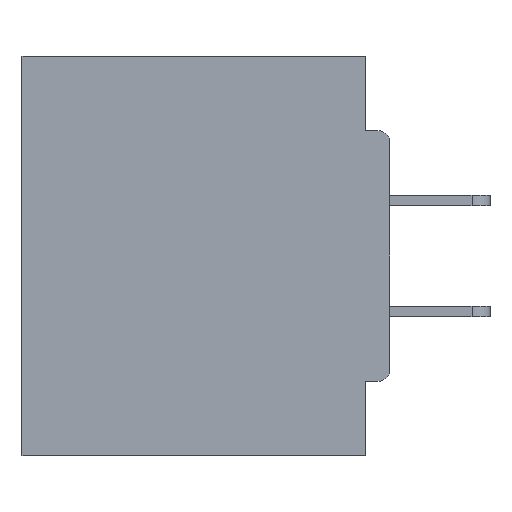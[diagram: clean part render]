
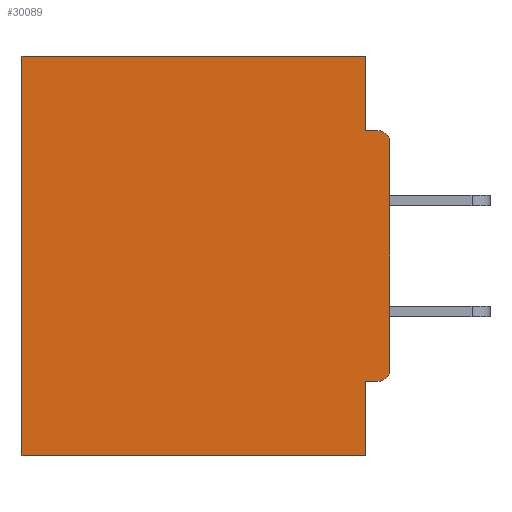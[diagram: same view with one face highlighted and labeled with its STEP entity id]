
A CAD part, left-side view. The second image highlights one B-rep face of the part: STEP entity #30089.
In plain terms, the highlighted planar face has unit normal (-1, 0, 0).
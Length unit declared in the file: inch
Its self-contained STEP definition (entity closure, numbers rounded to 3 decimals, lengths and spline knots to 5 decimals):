
#59 = ORIENTED_EDGE ( 'NONE', *, *, #22481, .F. ) ;
#153 = CIRCLE ( 'NONE', #36718, 0.015 ) ;
#462 = VERTEX_POINT ( 'NONE', #21627 ) ;
#936 = EDGE_CURVE ( 'NONE', #9909, #26018, #36658, .T. ) ;
#1723 = ORIENTED_EDGE ( 'NONE', *, *, #35162, .F. ) ;
#2313 = VECTOR ( 'NONE', #24132, 39.37008 ) ;
#2850 = CARTESIAN_POINT ( 'NONE',  ( 0.298, 0.015, -0.1085 ) ) ;
#4023 = DIRECTION ( 'NONE',  ( 0., 1., 0. ) ) ;
#4083 = CARTESIAN_POINT ( 'NONE',  ( 0.298, 0., 0. ) ) ;
#4333 = CIRCLE ( 'NONE', #4346, 0.015 ) ;
#4346 = AXIS2_PLACEMENT_3D ( 'NONE', #2850, #21541, #33391 ) ;
#4539 = ORIENTED_EDGE ( 'NONE', *, *, #19001, .T. ) ;
#4568 = LINE ( 'NONE', #33875, #5069 ) ;
#4732 = VECTOR ( 'NONE', #34768, 39.37008 ) ;
#4946 = FACE_OUTER_BOUND ( 'NONE', #10687, .T. ) ;
#5069 = VECTOR ( 'NONE', #34135, 39.37008 ) ;
#5492 = ORIENTED_EDGE ( 'NONE', *, *, #33387, .F. ) ;
#7512 = CARTESIAN_POINT ( 'NONE',  ( 0.298, 0.031, 0. ) ) ;
#7605 = AXIS2_PLACEMENT_3D ( 'NONE', #20560, #32809, #38469 ) ;
#7866 = VECTOR ( 'NONE', #4023, 39.37008 ) ;
#8174 = ORIENTED_EDGE ( 'NONE', *, *, #10169, .T. ) ;
#8887 = VECTOR ( 'NONE', #9446, 39.37008 ) ;
#9446 = DIRECTION ( 'NONE',  ( 0., 0., -1. ) ) ;
#9909 = VERTEX_POINT ( 'NONE', #7512 ) ;
#10169 = EDGE_CURVE ( 'NONE', #17332, #36294, #153, .T. ) ;
#10347 = DIRECTION ( 'NONE',  ( 0., 1., 0. ) ) ;
#10687 = EDGE_LOOP ( 'NONE', ( #37894, #35037, #59, #37771, #4539, #27794, #1723, #27116, #8174, #5492 ) ) ;
#12202 = VERTEX_POINT ( 'NONE', #34867 ) ;
#13095 = LINE ( 'NONE', #13332, #7866 ) ;
#13332 = CARTESIAN_POINT ( 'NONE',  ( 0.298, 0., -0.5 ) ) ;
#13822 = CARTESIAN_POINT ( 'NONE',  ( 0.298, 0., 0. ) ) ;
#13982 = EDGE_CURVE ( 'NONE', #462, #27365, #24177, .T. ) ;
#14369 = VECTOR ( 'NONE', #31480, 39.37008 ) ;
#15449 = CARTESIAN_POINT ( 'NONE',  ( 0.298, 0.46, 0. ) ) ;
#16356 = LINE ( 'NONE', #27222, #34872 ) ;
#17087 = LINE ( 'NONE', #13822, #4732 ) ;
#17332 = VERTEX_POINT ( 'NONE', #32124 ) ;
#19001 = EDGE_CURVE ( 'NONE', #26018, #21283, #16356, .T. ) ;
#19309 = VERTEX_POINT ( 'NONE', #31864 ) ;
#19492 = CARTESIAN_POINT ( 'NONE',  ( 0.298, 0., -0.4065 ) ) ;
#20560 = CARTESIAN_POINT ( 'NONE',  ( 0.298, 0., 0. ) ) ;
#21283 = VERTEX_POINT ( 'NONE', #28031 ) ;
#21541 = DIRECTION ( 'NONE',  ( -1., 0., 0. ) ) ;
#21627 = CARTESIAN_POINT ( 'NONE',  ( 0.298, 0.031, -0.0935 ) ) ;
#22481 = EDGE_CURVE ( 'NONE', #9909, #462, #32698, .T. ) ;
#24132 = DIRECTION ( 'NONE',  ( 0., -1., 0. ) ) ;
#24177 = LINE ( 'NONE', #38956, #2313 ) ;
#24803 = CARTESIAN_POINT ( 'NONE',  ( 0.298, 0., -0.1085 ) ) ;
#26018 = VERTEX_POINT ( 'NONE', #15449 ) ;
#26564 = LINE ( 'NONE', #19492, #35992 ) ;
#27116 = ORIENTED_EDGE ( 'NONE', *, *, #28807, .F. ) ;
#27187 = CARTESIAN_POINT ( 'NONE',  ( 0.298, 0.015, -0.3915 ) ) ;
#27222 = CARTESIAN_POINT ( 'NONE',  ( 0.298, 0.46, 0. ) ) ;
#27365 = VERTEX_POINT ( 'NONE', #33293 ) ;
#27794 = ORIENTED_EDGE ( 'NONE', *, *, #37872, .F. ) ;
#28031 = CARTESIAN_POINT ( 'NONE',  ( 0.298, 0.46, -0.5 ) ) ;
#28205 = CARTESIAN_POINT ( 'NONE',  ( 0.298, 0.031, -0.5 ) ) ;
#28807 = EDGE_CURVE ( 'NONE', #17332, #12202, #26564, .T. ) ;
#30089 = ADVANCED_FACE ( 'NONE', ( #4946 ), #32559, .F. ) ;
#30247 = CARTESIAN_POINT ( 'NONE',  ( 0.298, 0., -0.3915 ) ) ;
#31480 = DIRECTION ( 'NONE',  ( 0., 1., 0. ) ) ;
#31864 = CARTESIAN_POINT ( 'NONE',  ( 0.298, 0.031, -0.5 ) ) ;
#32124 = CARTESIAN_POINT ( 'NONE',  ( 0.298, 0.015, -0.4065 ) ) ;
#32431 = EDGE_CURVE ( 'NONE', #33738, #27365, #4333, .T. ) ;
#32559 = PLANE ( 'NONE',  #7605 ) ;
#32698 = LINE ( 'NONE', #28205, #8887 ) ;
#32809 = DIRECTION ( 'NONE',  ( 1., 0., 0. ) ) ;
#33009 = DIRECTION ( 'NONE',  ( 0., 0., -1. ) ) ;
#33293 = CARTESIAN_POINT ( 'NONE',  ( 0.298, 0.015, -0.0935 ) ) ;
#33387 = EDGE_CURVE ( 'NONE', #33738, #36294, #17087, .T. ) ;
#33391 = DIRECTION ( 'NONE',  ( 0., 0., -1. ) ) ;
#33738 = VERTEX_POINT ( 'NONE', #24803 ) ;
#33875 = CARTESIAN_POINT ( 'NONE',  ( 0.298, 0.031, -0.5 ) ) ;
#34135 = DIRECTION ( 'NONE',  ( 0., 0., -1. ) ) ;
#34768 = DIRECTION ( 'NONE',  ( 0., 0., -1. ) ) ;
#34867 = CARTESIAN_POINT ( 'NONE',  ( 0.298, 0.031, -0.4065 ) ) ;
#34872 = VECTOR ( 'NONE', #36202, 39.37008 ) ;
#35037 = ORIENTED_EDGE ( 'NONE', *, *, #13982, .F. ) ;
#35162 = EDGE_CURVE ( 'NONE', #12202, #19309, #4568, .T. ) ;
#35992 = VECTOR ( 'NONE', #10347, 39.37008 ) ;
#36202 = DIRECTION ( 'NONE',  ( 0., 0., -1. ) ) ;
#36294 = VERTEX_POINT ( 'NONE', #30247 ) ;
#36658 = LINE ( 'NONE', #4083, #14369 ) ;
#36718 = AXIS2_PLACEMENT_3D ( 'NONE', #27187, #39187, #33009 ) ;
#37771 = ORIENTED_EDGE ( 'NONE', *, *, #936, .T. ) ;
#37872 = EDGE_CURVE ( 'NONE', #19309, #21283, #13095, .T. ) ;
#37894 = ORIENTED_EDGE ( 'NONE', *, *, #32431, .T. ) ;
#38469 = DIRECTION ( 'NONE',  ( 0., 0., -1. ) ) ;
#38956 = CARTESIAN_POINT ( 'NONE',  ( 0.298, 0., -0.0935 ) ) ;
#39187 = DIRECTION ( 'NONE',  ( -1., 0., 0. ) ) ;
